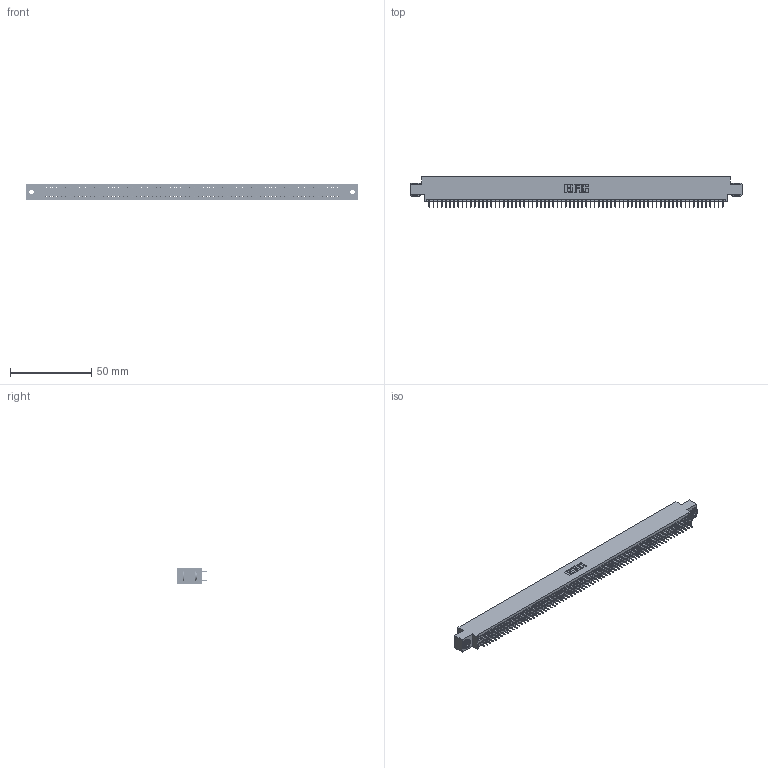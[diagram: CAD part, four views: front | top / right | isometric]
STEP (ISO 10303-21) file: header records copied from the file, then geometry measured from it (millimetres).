
FILE_DESCRIPTION (( 'STEP AP203' ), '1' );
FILE_NAME ('845-144-525-803.STEP', '2020-09-24T21:12:07', ( '' ), ( '' ), 'SwSTEP 2.0', 'SolidWorks 2020', '' );
FILE_SCHEMA (( 'CONFIG_CONTROL_DESIGN' ));
Length unit declared in the file: inch
Products named in the file (4): 845 Part_0.170 Offset - 0.156 Dia-TH; 845-144-525-803; 345-292-001_345-293-125; 345-250-002_345-250-002-102
Assembly tree (147 placements, depth 2):
  845-144-525-803
    845 Part_0.170 Offset - 0.156 Dia-TH
    345-292-001_345-293-125  x144
    345-250-002_345-250-002-102  x2
Bounding box: 204.09 x 18.72 x 9.4 mm (x, y, z)
Volume: 19772.9 mm3; surface area: 29442.8 mm2
Topology: 147 solids, 147 shells, 7944 faces, 22461 edges, 14394 vertices
Faces by surface type: plane 5710, cylinder 2226, cone 8
Entity records: 53310 total; most frequent: CARTESIAN_POINT 8883, ORIENTED_EDGE 8810, DIRECTION 7827, EDGE_CURVE 4405, VECTOR 3965, LINE 3965, VERTEX_POINT 2930, AXIS2_PLACEMENT_3D 1931
